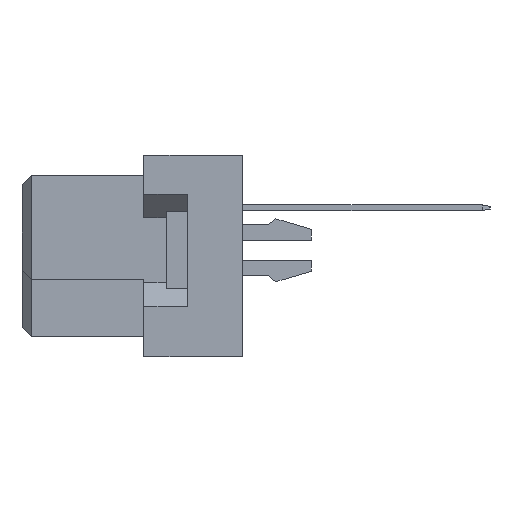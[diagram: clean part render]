
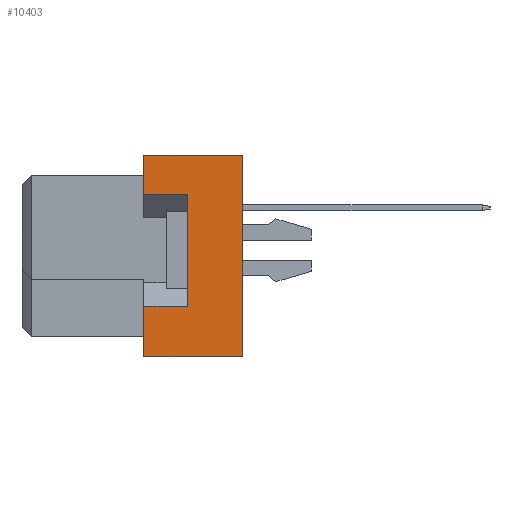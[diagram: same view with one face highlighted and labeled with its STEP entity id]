
A CAD part, left-side view. The second image highlights one B-rep face of the part: STEP entity #10403.
In plain terms, the highlighted planar face has unit normal (-1, 0, 0).
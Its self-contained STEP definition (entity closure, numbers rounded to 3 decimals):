
#220 = CARTESIAN_POINT ( 'NONE',  ( -47.5, -6.4, -2.65 ) ) ;
#455 = VERTEX_POINT ( 'NONE', #8612 ) ;
#935 = CARTESIAN_POINT ( 'NONE',  ( -47.5, -8.7, -2.65 ) ) ;
#999 = EDGE_CURVE ( 'NONE', #1638, #28599, #15859, .T. ) ;
#1638 = VERTEX_POINT ( 'NONE', #14790 ) ;
#1749 = DIRECTION ( 'NONE',  ( 0., 0., 1. ) ) ;
#2889 = EDGE_CURVE ( 'NONE', #10458, #20107, #11226, .T. ) ;
#3014 = VECTOR ( 'NONE', #12973, 1000. ) ;
#3383 = ORIENTED_EDGE ( 'NONE', *, *, #8893, .F. ) ;
#3451 = CARTESIAN_POINT ( 'NONE',  ( -47.5, -11.6, 5.3 ) ) ;
#3497 = VECTOR ( 'NONE', #12479, 1000. ) ;
#4407 = ORIENTED_EDGE ( 'NONE', *, *, #25011, .T. ) ;
#6161 = CARTESIAN_POINT ( 'NONE',  ( -47.5, -11.6, 5.3 ) ) ;
#8612 = CARTESIAN_POINT ( 'NONE',  ( -47.5, -6.4, 5.3 ) ) ;
#8893 = EDGE_CURVE ( 'NONE', #13330, #10453, #31501, .T. ) ;
#9195 = EDGE_CURVE ( 'NONE', #10453, #455, #15526, .T. ) ;
#9363 = FACE_OUTER_BOUND ( 'NONE', #11440, .T. ) ;
#9758 = CARTESIAN_POINT ( 'NONE',  ( -47.5, -6.4, 3.25 ) ) ;
#10403 = ADVANCED_FACE ( 'NONE', ( #9363 ), #24698, .T. ) ;
#10453 = VERTEX_POINT ( 'NONE', #9758 ) ;
#10458 = VERTEX_POINT ( 'NONE', #27694 ) ;
#10943 = EDGE_CURVE ( 'NONE', #33644, #28599, #16456, .T. ) ;
#11226 = LINE ( 'NONE', #23382, #11249 ) ;
#11249 = VECTOR ( 'NONE', #17403, 1000. ) ;
#11440 = EDGE_LOOP ( 'NONE', ( #24798, #27033, #20741, #36433, #4407, #19429, #3383, #24373 ) ) ;
#12020 = VECTOR ( 'NONE', #33162, 1000. ) ;
#12479 = DIRECTION ( 'NONE',  ( 0., 0., 1. ) ) ;
#12880 = CARTESIAN_POINT ( 'NONE',  ( -47.5, -6.4, -5.3 ) ) ;
#12973 = DIRECTION ( 'NONE',  ( 0., 1., 0. ) ) ;
#13330 = VERTEX_POINT ( 'NONE', #36389 ) ;
#13354 = CARTESIAN_POINT ( 'NONE',  ( -47.5, -8.7, 3.25 ) ) ;
#14790 = CARTESIAN_POINT ( 'NONE',  ( -47.5, -6.4, -5.3 ) ) ;
#15411 = LINE ( 'NONE', #3451, #12020 ) ;
#15526 = LINE ( 'NONE', #27100, #16613 ) ;
#15859 = LINE ( 'NONE', #12880, #3497 ) ;
#16456 = LINE ( 'NONE', #31022, #21719 ) ;
#16613 = VECTOR ( 'NONE', #39261, 1000. ) ;
#16701 = CARTESIAN_POINT ( 'NONE',  ( -47.5, -8.7, -2.65 ) ) ;
#17403 = DIRECTION ( 'NONE',  ( 0., 0., 1. ) ) ;
#18136 = DIRECTION ( 'NONE',  ( -1., 0., 0. ) ) ;
#19065 = CARTESIAN_POINT ( 'NONE',  ( -47.5, -11.6, -5.3 ) ) ;
#19429 = ORIENTED_EDGE ( 'NONE', *, *, #9195, .F. ) ;
#20107 = VERTEX_POINT ( 'NONE', #28856 ) ;
#20741 = ORIENTED_EDGE ( 'NONE', *, *, #32450, .F. ) ;
#21549 = VECTOR ( 'NONE', #1749, 1000. ) ;
#21719 = VECTOR ( 'NONE', #28032, 1000. ) ;
#23382 = CARTESIAN_POINT ( 'NONE',  ( -47.5, -11.6, 5.3 ) ) ;
#24373 = ORIENTED_EDGE ( 'NONE', *, *, #37677, .F. ) ;
#24698 = PLANE ( 'NONE',  #38889 ) ;
#24798 = ORIENTED_EDGE ( 'NONE', *, *, #10943, .T. ) ;
#25011 = EDGE_CURVE ( 'NONE', #20107, #455, #15411, .T. ) ;
#27033 = ORIENTED_EDGE ( 'NONE', *, *, #999, .F. ) ;
#27100 = CARTESIAN_POINT ( 'NONE',  ( -47.5, -6.4, -5.3 ) ) ;
#27694 = CARTESIAN_POINT ( 'NONE',  ( -47.5, -11.6, -5.3 ) ) ;
#28032 = DIRECTION ( 'NONE',  ( 0., 1., 0. ) ) ;
#28039 = DIRECTION ( 'NONE',  ( 0., 1., 0. ) ) ;
#28599 = VERTEX_POINT ( 'NONE', #220 ) ;
#28719 = VECTOR ( 'NONE', #28039, 1000. ) ;
#28856 = CARTESIAN_POINT ( 'NONE',  ( -47.5, -11.6, 5.3 ) ) ;
#31022 = CARTESIAN_POINT ( 'NONE',  ( -47.5, -8.7, -2.65 ) ) ;
#31501 = LINE ( 'NONE', #13354, #3014 ) ;
#32450 = EDGE_CURVE ( 'NONE', #10458, #1638, #37020, .T. ) ;
#33162 = DIRECTION ( 'NONE',  ( 0., 1., 0. ) ) ;
#33644 = VERTEX_POINT ( 'NONE', #935 ) ;
#34643 = LINE ( 'NONE', #16701, #21549 ) ;
#36389 = CARTESIAN_POINT ( 'NONE',  ( -47.5, -8.7, 3.25 ) ) ;
#36433 = ORIENTED_EDGE ( 'NONE', *, *, #2889, .T. ) ;
#36861 = DIRECTION ( 'NONE',  ( 0., 0., 1. ) ) ;
#37020 = LINE ( 'NONE', #19065, #28719 ) ;
#37677 = EDGE_CURVE ( 'NONE', #33644, #13330, #34643, .T. ) ;
#38889 = AXIS2_PLACEMENT_3D ( 'NONE', #6161, #18136, #36861 ) ;
#39261 = DIRECTION ( 'NONE',  ( 0., 0., 1. ) ) ;
